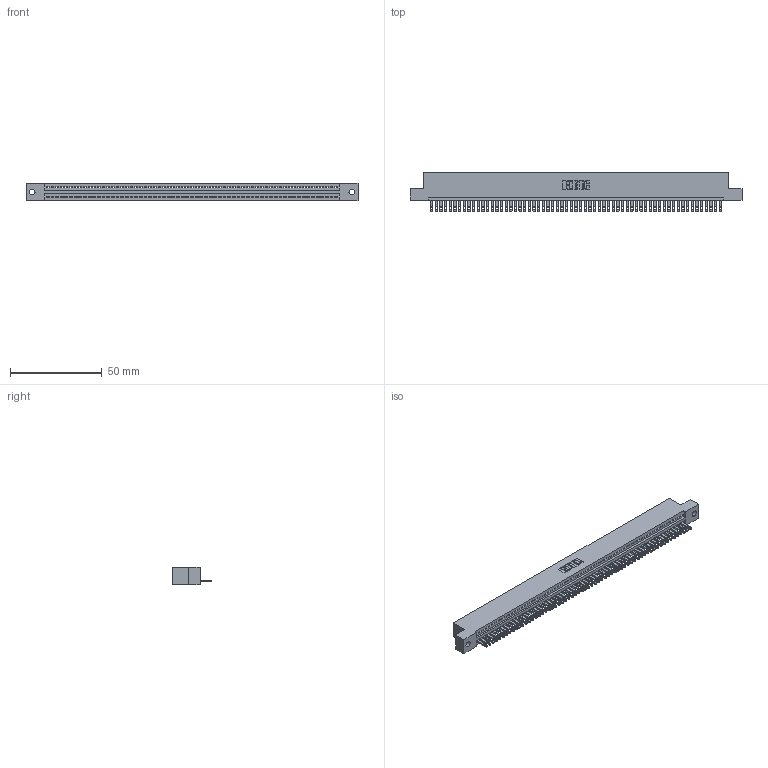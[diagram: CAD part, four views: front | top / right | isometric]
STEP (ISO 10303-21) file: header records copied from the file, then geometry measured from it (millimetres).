
FILE_DESCRIPTION (( 'STEP AP203' ), '1' );
FILE_NAME ('345-063-500-102.STEP', '2019-10-11T08:11:57', ( '' ), ( '' ), 'SwSTEP 2.0', 'SolidWorks 2016', '' );
FILE_SCHEMA (( 'CONFIG_CONTROL_DESIGN' ));
Length unit declared in the file: inch
Products named in the file (3): 345-292-001_345-293-100; 345 Part_Flush Mounting Lugs - 0.128 Dia; 345-063-500-102
Assembly tree (64 placements, depth 2):
  345-063-500-102
    345 Part_Flush Mounting Lugs - 0.128 Dia
    345-292-001_345-293-100  x63
Bounding box: 181.23 x 21.51 x 9.4 mm (x, y, z)
Volume: 17387.6 mm3; surface area: 23262 mm2
Topology: 64 solids, 64 shells, 3528 faces, 10925 edges, 7282 vertices
Faces by surface type: plane 2222, cylinder 1306
Entity records: 44521 total; most frequent: CARTESIAN_POINT 7717, ORIENTED_EDGE 7714, DIRECTION 6711, EDGE_CURVE 3857, LINE 3469, VECTOR 3469, VERTEX_POINT 2570, AXIS2_PLACEMENT_3D 1621
